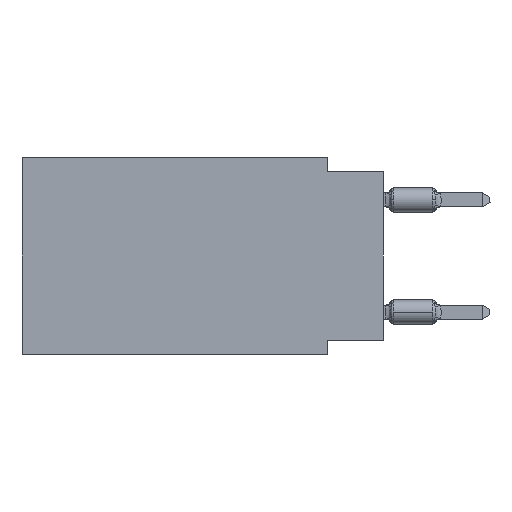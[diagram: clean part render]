
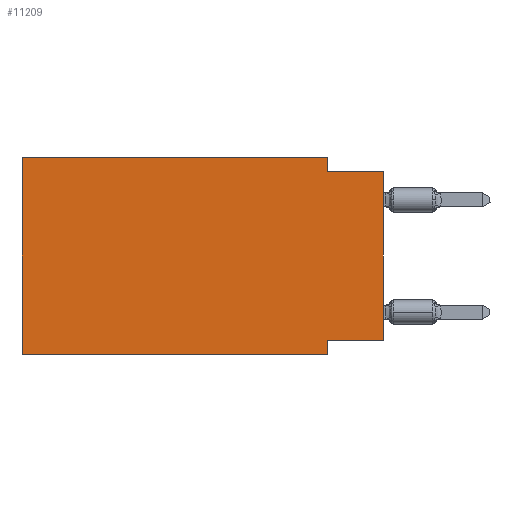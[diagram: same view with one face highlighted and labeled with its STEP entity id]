
A CAD part, left-side view. The second image highlights one B-rep face of the part: STEP entity #11209.
In plain terms, the highlighted planar face has unit normal (-1, 0, 0).
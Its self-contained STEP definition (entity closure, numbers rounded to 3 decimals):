
#776 = VERTEX_POINT ( 'NONE', #20078 ) ;
#1828 = AXIS2_PLACEMENT_3D ( 'NONE', #54929, #13845, #22648 ) ;
#3329 = CARTESIAN_POINT ( 'NONE',  ( 0., 0., -8.255 ) ) ;
#3760 = LINE ( 'NONE', #12239, #30297 ) ;
#4771 = LINE ( 'NONE', #27788, #21943 ) ;
#5412 = ORIENTED_EDGE ( 'NONE', *, *, #34345, .F. ) ;
#6979 = DIRECTION ( 'NONE',  ( 0., 0., -1. ) ) ;
#7491 = EDGE_CURVE ( 'NONE', #31513, #776, #23182, .T. ) ;
#7691 = VECTOR ( 'NONE', #50294, 1000. ) ;
#10080 = VECTOR ( 'NONE', #36950, 1000. ) ;
#11209 = ADVANCED_FACE ( 'NONE', ( #17816 ), #13560, .F. ) ;
#12239 = CARTESIAN_POINT ( 'NONE',  ( 0., 16.383, 0. ) ) ;
#12468 = CARTESIAN_POINT ( 'NONE',  ( 0., 2.54, 0. ) ) ;
#13082 = ORIENTED_EDGE ( 'NONE', *, *, #22265, .F. ) ;
#13376 = EDGE_CURVE ( 'NONE', #57796, #28107, #4771, .T. ) ;
#13560 = PLANE ( 'NONE',  #1828 ) ;
#13845 = DIRECTION ( 'NONE',  ( 1., 0., 0. ) ) ;
#14035 = LINE ( 'NONE', #24011, #7691 ) ;
#16094 = LINE ( 'NONE', #53539, #56318 ) ;
#16215 = CARTESIAN_POINT ( 'NONE',  ( 0., 2.54, -8.255 ) ) ;
#17238 = CARTESIAN_POINT ( 'NONE',  ( 0., 2.54, -8.89 ) ) ;
#17816 = FACE_OUTER_BOUND ( 'NONE', #57830, .T. ) ;
#18544 = LINE ( 'NONE', #51153, #10080 ) ;
#19236 = CARTESIAN_POINT ( 'NONE',  ( 0., 16.383, -8.89 ) ) ;
#20078 = CARTESIAN_POINT ( 'NONE',  ( 0., 2.54, -8.89 ) ) ;
#21128 = ORIENTED_EDGE ( 'NONE', *, *, #13376, .F. ) ;
#21190 = ORIENTED_EDGE ( 'NONE', *, *, #36941, .F. ) ;
#21943 = VECTOR ( 'NONE', #32289, 1000. ) ;
#22265 = EDGE_CURVE ( 'NONE', #31513, #49598, #14035, .T. ) ;
#22648 = DIRECTION ( 'NONE',  ( 0., 0., -1. ) ) ;
#23182 = LINE ( 'NONE', #19236, #57444 ) ;
#24011 = CARTESIAN_POINT ( 'NONE',  ( 0., 16.383, 0. ) ) ;
#27788 = CARTESIAN_POINT ( 'NONE',  ( 0., 0., -0.635 ) ) ;
#28107 = VERTEX_POINT ( 'NONE', #55399 ) ;
#30297 = VECTOR ( 'NONE', #30697, 1000. ) ;
#30697 = DIRECTION ( 'NONE',  ( 0., -1., 0. ) ) ;
#31124 = ORIENTED_EDGE ( 'NONE', *, *, #34725, .F. ) ;
#31513 = VERTEX_POINT ( 'NONE', #52866 ) ;
#32289 = DIRECTION ( 'NONE',  ( 0., -1., 0. ) ) ;
#34345 = EDGE_CURVE ( 'NONE', #57866, #57796, #16094, .T. ) ;
#34725 = EDGE_CURVE ( 'NONE', #43763, #42521, #46270, .T. ) ;
#35645 = DIRECTION ( 'NONE',  ( 0., 0., -1. ) ) ;
#36941 = EDGE_CURVE ( 'NONE', #42521, #776, #54068, .T. ) ;
#36950 = DIRECTION ( 'NONE',  ( 0., 0., 1. ) ) ;
#38688 = ORIENTED_EDGE ( 'NONE', *, *, #7491, .T. ) ;
#40319 = ORIENTED_EDGE ( 'NONE', *, *, #41959, .T. ) ;
#41100 = VECTOR ( 'NONE', #35645, 1000. ) ;
#41959 = EDGE_CURVE ( 'NONE', #43763, #28107, #18544, .T. ) ;
#42521 = VERTEX_POINT ( 'NONE', #16215 ) ;
#42640 = CARTESIAN_POINT ( 'NONE',  ( 0., 0., -8.255 ) ) ;
#43189 = ORIENTED_EDGE ( 'NONE', *, *, #59141, .F. ) ;
#43763 = VERTEX_POINT ( 'NONE', #3329 ) ;
#46270 = LINE ( 'NONE', #42640, #50583 ) ;
#46864 = DIRECTION ( 'NONE',  ( 0., 1., 0. ) ) ;
#49598 = VERTEX_POINT ( 'NONE', #54996 ) ;
#50294 = DIRECTION ( 'NONE',  ( 0., 0., 1. ) ) ;
#50583 = VECTOR ( 'NONE', #46864, 1000. ) ;
#51153 = CARTESIAN_POINT ( 'NONE',  ( 0., 0., 0. ) ) ;
#52866 = CARTESIAN_POINT ( 'NONE',  ( 0., 16.383, -8.89 ) ) ;
#53539 = CARTESIAN_POINT ( 'NONE',  ( 0., 2.54, 0. ) ) ;
#54068 = LINE ( 'NONE', #17238, #41100 ) ;
#54157 = CARTESIAN_POINT ( 'NONE',  ( 0., 2.54, -0.635 ) ) ;
#54929 = CARTESIAN_POINT ( 'NONE',  ( 0., 16.383, 0. ) ) ;
#54996 = CARTESIAN_POINT ( 'NONE',  ( 0., 16.383, 0. ) ) ;
#55164 = DIRECTION ( 'NONE',  ( 0., -1., 0. ) ) ;
#55399 = CARTESIAN_POINT ( 'NONE',  ( 0., 0., -0.635 ) ) ;
#56318 = VECTOR ( 'NONE', #6979, 1000. ) ;
#57444 = VECTOR ( 'NONE', #55164, 1000. ) ;
#57796 = VERTEX_POINT ( 'NONE', #54157 ) ;
#57830 = EDGE_LOOP ( 'NONE', ( #40319, #21128, #5412, #43189, #13082, #38688, #21190, #31124 ) ) ;
#57866 = VERTEX_POINT ( 'NONE', #12468 ) ;
#59141 = EDGE_CURVE ( 'NONE', #49598, #57866, #3760, .T. ) ;
